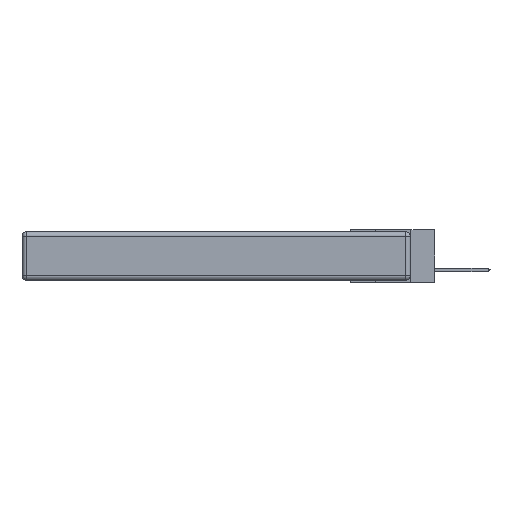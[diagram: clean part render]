
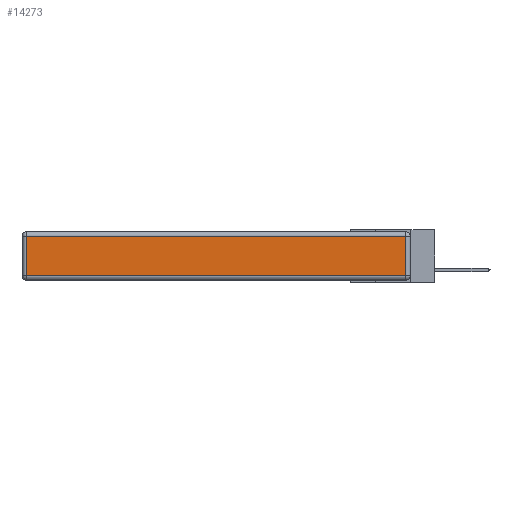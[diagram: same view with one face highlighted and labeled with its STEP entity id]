
A CAD part, left-side view. The second image highlights one B-rep face of the part: STEP entity #14273.
In plain terms, the highlighted planar face has unit normal (-1, 0, 0).
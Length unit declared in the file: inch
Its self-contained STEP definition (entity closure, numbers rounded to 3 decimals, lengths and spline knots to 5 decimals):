
#34 = VERTEX_POINT ( 'NONE', #12431 ) ;
#100 = EDGE_LOOP ( 'NONE', ( #1419, #15568, #13624, #18026 ) ) ;
#731 = LINE ( 'NONE', #12982, #12435 ) ;
#1419 = ORIENTED_EDGE ( 'NONE', *, *, #15567, .T. ) ;
#2459 = DIRECTION ( 'NONE',  ( 0., 0., 1. ) ) ;
#3743 = CARTESIAN_POINT ( 'NONE',  ( 0., 2.72, -0.343 ) ) ;
#4461 = LINE ( 'NONE', #3743, #14083 ) ;
#5413 = CARTESIAN_POINT ( 'NONE',  ( 0., 2.75, -0.03 ) ) ;
#5497 = DIRECTION ( 'NONE',  ( 0., -1., 0. ) ) ;
#5850 = VERTEX_POINT ( 'NONE', #15735 ) ;
#9821 = DIRECTION ( 'NONE',  ( 0., 0., -1. ) ) ;
#10316 = CARTESIAN_POINT ( 'NONE',  ( 0., 0.03, -0.313 ) ) ;
#10706 = VERTEX_POINT ( 'NONE', #10316 ) ;
#11278 = CARTESIAN_POINT ( 'NONE',  ( 0., 0., -0.343 ) ) ;
#11335 = FACE_OUTER_BOUND ( 'NONE', #100, .T. ) ;
#11792 = VERTEX_POINT ( 'NONE', #19264 ) ;
#12019 = LINE ( 'NONE', #16087, #16251 ) ;
#12431 = CARTESIAN_POINT ( 'NONE',  ( 0., 2.72, -0.313 ) ) ;
#12435 = VECTOR ( 'NONE', #5497, 39.37008 ) ;
#12941 = DIRECTION ( 'NONE',  ( 0., 0., 1. ) ) ;
#12982 = CARTESIAN_POINT ( 'NONE',  ( 0., 0., -0.313 ) ) ;
#13207 = LINE ( 'NONE', #5413, #13898 ) ;
#13624 = ORIENTED_EDGE ( 'NONE', *, *, #14234, .T. ) ;
#13898 = VECTOR ( 'NONE', #14484, 39.37008 ) ;
#14083 = VECTOR ( 'NONE', #9821, 39.37008 ) ;
#14234 = EDGE_CURVE ( 'NONE', #5850, #11792, #13207, .T. ) ;
#14273 = ADVANCED_FACE ( 'NONE', ( #11335 ), #17426, .T. ) ;
#14484 = DIRECTION ( 'NONE',  ( 0., 1., 0. ) ) ;
#15567 = EDGE_CURVE ( 'NONE', #34, #10706, #731, .T. ) ;
#15568 = ORIENTED_EDGE ( 'NONE', *, *, #17249, .T. ) ;
#15735 = CARTESIAN_POINT ( 'NONE',  ( 0., 0.03, -0.03 ) ) ;
#15792 = DIRECTION ( 'NONE',  ( -1., 0., 0. ) ) ;
#16087 = CARTESIAN_POINT ( 'NONE',  ( 0., 0.03, -0.343 ) ) ;
#16251 = VECTOR ( 'NONE', #12941, 39.37008 ) ;
#17249 = EDGE_CURVE ( 'NONE', #10706, #5850, #12019, .T. ) ;
#17426 = PLANE ( 'NONE',  #18102 ) ;
#18026 = ORIENTED_EDGE ( 'NONE', *, *, #18139, .T. ) ;
#18102 = AXIS2_PLACEMENT_3D ( 'NONE', #11278, #15792, #2459 ) ;
#18139 = EDGE_CURVE ( 'NONE', #11792, #34, #4461, .T. ) ;
#19264 = CARTESIAN_POINT ( 'NONE',  ( 0., 2.72, -0.03 ) ) ;
